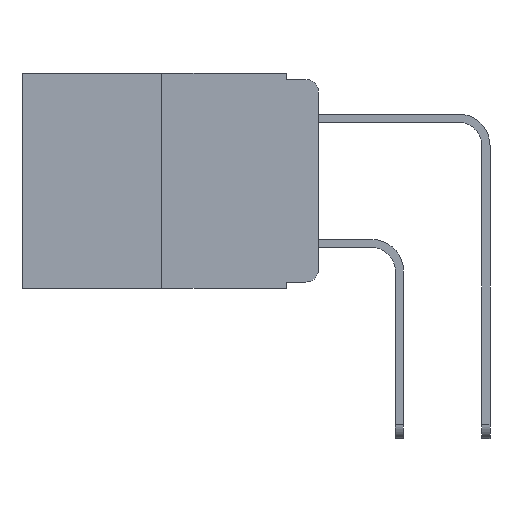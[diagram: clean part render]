
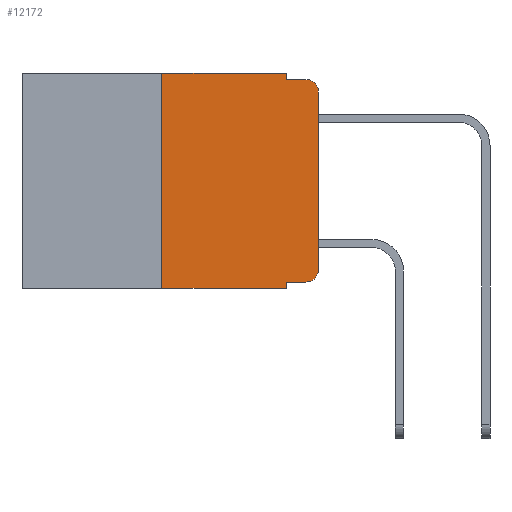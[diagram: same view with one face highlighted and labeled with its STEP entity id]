
A CAD part, left-side view. The second image highlights one B-rep face of the part: STEP entity #12172.
In plain terms, the highlighted planar face has unit normal (-1, 0, 0).
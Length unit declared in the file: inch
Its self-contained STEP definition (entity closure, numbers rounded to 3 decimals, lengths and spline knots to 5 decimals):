
#54 = DIRECTION ( 'NONE',  ( 0., -1., 0. ) ) ;
#499 = ORIENTED_EDGE ( 'NONE', *, *, #13059, .T. ) ;
#627 = CARTESIAN_POINT ( 'NONE',  ( 0., 0.02, -0.313 ) ) ;
#744 = CARTESIAN_POINT ( 'NONE',  ( 0., 0.02, -0.01 ) ) ;
#820 = LINE ( 'NONE', #2813, #3815 ) ;
#1069 = DIRECTION ( 'NONE',  ( 0., 0., 1. ) ) ;
#1149 = ORIENTED_EDGE ( 'NONE', *, *, #6412, .F. ) ;
#1449 = EDGE_CURVE ( 'NONE', #1817, #7054, #3596, .T. ) ;
#1760 = DIRECTION ( 'NONE',  ( 0., 0., -1. ) ) ;
#1817 = VERTEX_POINT ( 'NONE', #8702 ) ;
#1828 = CARTESIAN_POINT ( 'NONE',  ( 0., 0.051, -0.333 ) ) ;
#1901 = LINE ( 'NONE', #12805, #2253 ) ;
#1935 = ORIENTED_EDGE ( 'NONE', *, *, #4689, .T. ) ;
#2151 = VERTEX_POINT ( 'NONE', #10805 ) ;
#2253 = VECTOR ( 'NONE', #54, 39.37008 ) ;
#2541 = ORIENTED_EDGE ( 'NONE', *, *, #11291, .F. ) ;
#2548 = CARTESIAN_POINT ( 'NONE',  ( 0., 0.473, 0. ) ) ;
#2727 = ORIENTED_EDGE ( 'NONE', *, *, #7272, .F. ) ;
#2769 = LINE ( 'NONE', #1828, #5018 ) ;
#2798 = CIRCLE ( 'NONE', #3769, 0.02 ) ;
#2813 = CARTESIAN_POINT ( 'NONE',  ( 0., 0.25, 0. ) ) ;
#2858 = DIRECTION ( 'NONE',  ( 0., 0., 1. ) ) ;
#2911 = AXIS2_PLACEMENT_3D ( 'NONE', #4925, #12205, #5990 ) ;
#3372 = CARTESIAN_POINT ( 'NONE',  ( 0., 0.473, 0. ) ) ;
#3596 = LINE ( 'NONE', #11174, #12284 ) ;
#3761 = ORIENTED_EDGE ( 'NONE', *, *, #4999, .T. ) ;
#3769 = AXIS2_PLACEMENT_3D ( 'NONE', #627, #8201, #1760 ) ;
#3784 = VECTOR ( 'NONE', #5112, 39.37008 ) ;
#3815 = VECTOR ( 'NONE', #2858, 39.37008 ) ;
#3941 = ORIENTED_EDGE ( 'NONE', *, *, #5864, .T. ) ;
#3988 = AXIS2_PLACEMENT_3D ( 'NONE', #3372, #4465, #11778 ) ;
#4068 = CARTESIAN_POINT ( 'NONE',  ( 0., 0., -0.313 ) ) ;
#4072 = VECTOR ( 'NONE', #8305, 39.37008 ) ;
#4110 = LINE ( 'NONE', #6118, #3784 ) ;
#4258 = VERTEX_POINT ( 'NONE', #9461 ) ;
#4439 = VECTOR ( 'NONE', #11030, 39.37008 ) ;
#4465 = DIRECTION ( 'NONE',  ( 1., 0., 0. ) ) ;
#4689 = EDGE_CURVE ( 'NONE', #2151, #7278, #2798, .T. ) ;
#4925 = CARTESIAN_POINT ( 'NONE',  ( 0., 0.02, -0.03 ) ) ;
#4947 = CARTESIAN_POINT ( 'NONE',  ( 0., 0.25, -0.343 ) ) ;
#4999 = EDGE_CURVE ( 'NONE', #8813, #4258, #1901, .T. ) ;
#5018 = VECTOR ( 'NONE', #5168, 39.37008 ) ;
#5112 = DIRECTION ( 'NONE',  ( 0., 0., -1. ) ) ;
#5168 = DIRECTION ( 'NONE',  ( 0., -1., 0. ) ) ;
#5864 = EDGE_CURVE ( 'NONE', #6623, #7273, #13100, .T. ) ;
#5949 = EDGE_CURVE ( 'NONE', #9453, #4258, #4110, .T. ) ;
#5990 = DIRECTION ( 'NONE',  ( 0., 0., -1. ) ) ;
#6118 = CARTESIAN_POINT ( 'NONE',  ( 0., 0.051, 0. ) ) ;
#6285 = ORIENTED_EDGE ( 'NONE', *, *, #5949, .F. ) ;
#6412 = EDGE_CURVE ( 'NONE', #13411, #1817, #7270, .T. ) ;
#6623 = VERTEX_POINT ( 'NONE', #10331 ) ;
#6932 = LINE ( 'NONE', #12427, #4072 ) ;
#7054 = VERTEX_POINT ( 'NONE', #10001 ) ;
#7270 = LINE ( 'NONE', #2548, #4439 ) ;
#7272 = EDGE_CURVE ( 'NONE', #7054, #7273, #6932, .T. ) ;
#7273 = VERTEX_POINT ( 'NONE', #744 ) ;
#7278 = VERTEX_POINT ( 'NONE', #4068 ) ;
#7589 = ORIENTED_EDGE ( 'NONE', *, *, #12128, .T. ) ;
#7833 = FACE_OUTER_BOUND ( 'NONE', #10887, .T. ) ;
#8201 = DIRECTION ( 'NONE',  ( -1., 0., 0. ) ) ;
#8305 = DIRECTION ( 'NONE',  ( 0., -1., 0. ) ) ;
#8702 = CARTESIAN_POINT ( 'NONE',  ( 0., 0.051, 0. ) ) ;
#8813 = VERTEX_POINT ( 'NONE', #4947 ) ;
#9453 = VERTEX_POINT ( 'NONE', #13199 ) ;
#9461 = CARTESIAN_POINT ( 'NONE',  ( 0., 0.051, -0.343 ) ) ;
#9847 = CARTESIAN_POINT ( 'NONE',  ( 0., 0.25, 0. ) ) ;
#9856 = ORIENTED_EDGE ( 'NONE', *, *, #1449, .F. ) ;
#10001 = CARTESIAN_POINT ( 'NONE',  ( 0., 0.051, -0.01 ) ) ;
#10331 = CARTESIAN_POINT ( 'NONE',  ( 0., 0., -0.03 ) ) ;
#10748 = PLANE ( 'NONE',  #3988 ) ;
#10805 = CARTESIAN_POINT ( 'NONE',  ( 0., 0.02, -0.333 ) ) ;
#10887 = EDGE_LOOP ( 'NONE', ( #7589, #3941, #2727, #9856, #1149, #2541, #3761, #6285, #499, #1935 ) ) ;
#10918 = VECTOR ( 'NONE', #1069, 39.37008 ) ;
#11030 = DIRECTION ( 'NONE',  ( 0., -1., 0. ) ) ;
#11174 = CARTESIAN_POINT ( 'NONE',  ( 0., 0.051, 0. ) ) ;
#11212 = DIRECTION ( 'NONE',  ( 0., 0., -1. ) ) ;
#11291 = EDGE_CURVE ( 'NONE', #8813, #13411, #820, .T. ) ;
#11778 = DIRECTION ( 'NONE',  ( 0., 0., -1. ) ) ;
#12128 = EDGE_CURVE ( 'NONE', #7278, #6623, #13627, .T. ) ;
#12172 = ADVANCED_FACE ( 'NONE', ( #7833 ), #10748, .F. ) ;
#12205 = DIRECTION ( 'NONE',  ( -1., 0., 0. ) ) ;
#12284 = VECTOR ( 'NONE', #11212, 39.37008 ) ;
#12427 = CARTESIAN_POINT ( 'NONE',  ( 0., 0.051, -0.01 ) ) ;
#12726 = CARTESIAN_POINT ( 'NONE',  ( 0., 0., 0. ) ) ;
#12805 = CARTESIAN_POINT ( 'NONE',  ( 0., 0.473, -0.343 ) ) ;
#13059 = EDGE_CURVE ( 'NONE', #9453, #2151, #2769, .T. ) ;
#13100 = CIRCLE ( 'NONE', #2911, 0.02 ) ;
#13199 = CARTESIAN_POINT ( 'NONE',  ( 0., 0.051, -0.333 ) ) ;
#13411 = VERTEX_POINT ( 'NONE', #9847 ) ;
#13627 = LINE ( 'NONE', #12726, #10918 ) ;
